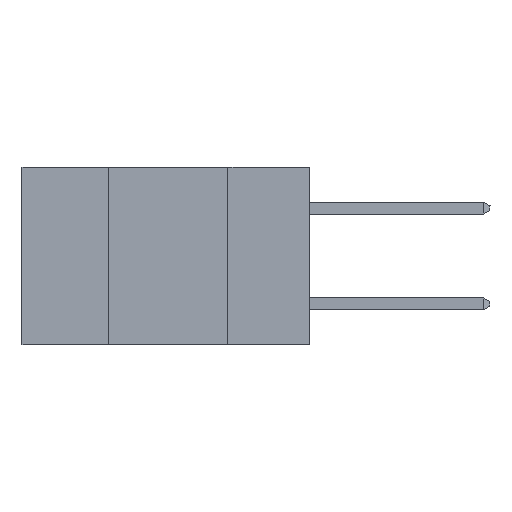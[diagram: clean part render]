
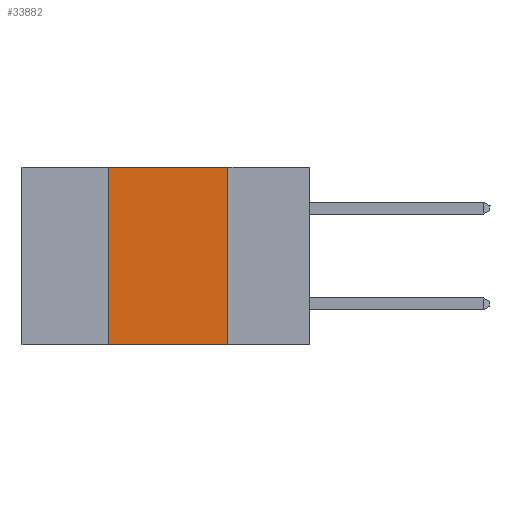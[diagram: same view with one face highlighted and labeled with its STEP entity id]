
A CAD part, left-side view. The second image highlights one B-rep face of the part: STEP entity #33882.
In plain terms, the highlighted planar face has unit normal (-1, 0, 0).
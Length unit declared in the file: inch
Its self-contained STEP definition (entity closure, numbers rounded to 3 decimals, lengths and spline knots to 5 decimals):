
#2767 = DIRECTION ( 'NONE',  ( 0., -1., 0. ) ) ;
#2898 = VERTEX_POINT ( 'NONE', #35667 ) ;
#3427 = DIRECTION ( 'NONE',  ( 0., 0., -1. ) ) ;
#5957 = CARTESIAN_POINT ( 'NONE',  ( 0., 0.6, 0. ) ) ;
#7215 = ORIENTED_EDGE ( 'NONE', *, *, #33140, .F. ) ;
#7253 = CARTESIAN_POINT ( 'NONE',  ( 0., 0.42, 0. ) ) ;
#7563 = VERTEX_POINT ( 'NONE', #16629 ) ;
#7793 = VECTOR ( 'NONE', #20156, 39.37008 ) ;
#9547 = CARTESIAN_POINT ( 'NONE',  ( 0., 0.6, -0.37 ) ) ;
#10036 = CARTESIAN_POINT ( 'NONE',  ( 0., 0.42, -0.37 ) ) ;
#10853 = DIRECTION ( 'NONE',  ( 0., 0., -1. ) ) ;
#14252 = CARTESIAN_POINT ( 'NONE',  ( 0., 0.17, 0. ) ) ;
#16629 = CARTESIAN_POINT ( 'NONE',  ( 0., 0.17, -0.37 ) ) ;
#17190 = LINE ( 'NONE', #9547, #7793 ) ;
#19037 = EDGE_CURVE ( 'NONE', #26399, #23182, #33380, .T. ) ;
#20156 = DIRECTION ( 'NONE',  ( 0., -1., 0. ) ) ;
#20954 = CARTESIAN_POINT ( 'NONE',  ( 0., 0.6, 0. ) ) ;
#22496 = EDGE_CURVE ( 'NONE', #26399, #7563, #17190, .T. ) ;
#22931 = VECTOR ( 'NONE', #2767, 39.37008 ) ;
#23182 = VERTEX_POINT ( 'NONE', #44624 ) ;
#24491 = DIRECTION ( 'NONE',  ( 1., 0., 0. ) ) ;
#26399 = VERTEX_POINT ( 'NONE', #10036 ) ;
#28143 = ORIENTED_EDGE ( 'NONE', *, *, #22496, .T. ) ;
#32021 = ORIENTED_EDGE ( 'NONE', *, *, #41884, .F. ) ;
#32134 = FACE_OUTER_BOUND ( 'NONE', #34447, .T. ) ;
#33140 = EDGE_CURVE ( 'NONE', #2898, #7563, #38222, .T. ) ;
#33380 = LINE ( 'NONE', #7253, #41564 ) ;
#33882 = ADVANCED_FACE ( 'NONE', ( #32134 ), #41963, .F. ) ;
#34447 = EDGE_LOOP ( 'NONE', ( #7215, #32021, #38612, #28143 ) ) ;
#35367 = DIRECTION ( 'NONE',  ( 0., 0., 1. ) ) ;
#35556 = LINE ( 'NONE', #5957, #22931 ) ;
#35667 = CARTESIAN_POINT ( 'NONE',  ( 0., 0.17, 0. ) ) ;
#37143 = VECTOR ( 'NONE', #10853, 39.37008 ) ;
#38222 = LINE ( 'NONE', #14252, #37143 ) ;
#38612 = ORIENTED_EDGE ( 'NONE', *, *, #19037, .F. ) ;
#41564 = VECTOR ( 'NONE', #35367, 39.37008 ) ;
#41884 = EDGE_CURVE ( 'NONE', #23182, #2898, #35556, .T. ) ;
#41963 = PLANE ( 'NONE',  #44036 ) ;
#44036 = AXIS2_PLACEMENT_3D ( 'NONE', #20954, #24491, #3427 ) ;
#44624 = CARTESIAN_POINT ( 'NONE',  ( 0., 0.42, 0. ) ) ;
